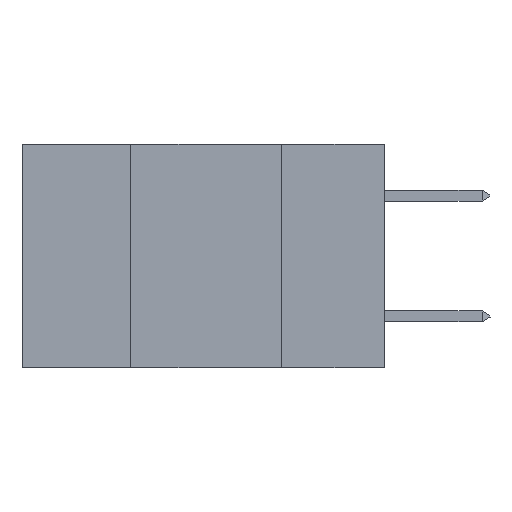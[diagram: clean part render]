
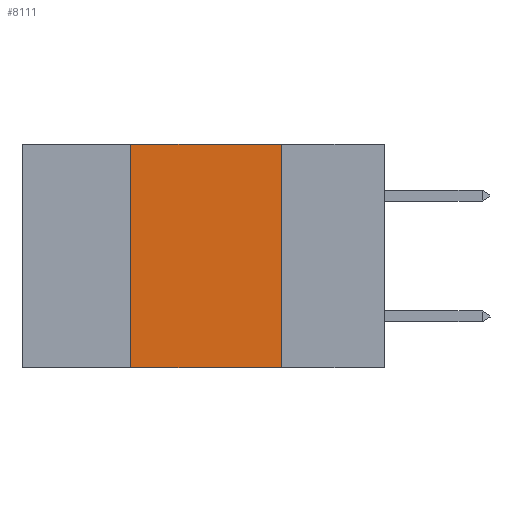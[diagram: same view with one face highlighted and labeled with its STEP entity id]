
A CAD part, left-side view. The second image highlights one B-rep face of the part: STEP entity #8111.
In plain terms, the highlighted planar face has unit normal (-1, 0, 0).
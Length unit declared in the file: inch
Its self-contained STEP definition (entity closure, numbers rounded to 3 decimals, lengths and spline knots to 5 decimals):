
#73 = CARTESIAN_POINT ( 'NONE',  ( 0., 0.17, 0. ) ) ;
#305 = ORIENTED_EDGE ( 'NONE', *, *, #475, .T. ) ;
#368 = CARTESIAN_POINT ( 'NONE',  ( 0., 0.17, 0. ) ) ;
#475 = EDGE_CURVE ( 'NONE', #9126, #8921, #4861, .T. ) ;
#551 = DIRECTION ( 'NONE',  ( 0., 0., 1. ) ) ;
#1289 = CARTESIAN_POINT ( 'NONE',  ( 0., 0.42, 0. ) ) ;
#1982 = DIRECTION ( 'NONE',  ( 0., 0., -1. ) ) ;
#2346 = VECTOR ( 'NONE', #6674, 39.37008 ) ;
#2566 = VERTEX_POINT ( 'NONE', #73 ) ;
#2651 = FACE_OUTER_BOUND ( 'NONE', #8831, .T. ) ;
#2859 = VECTOR ( 'NONE', #6045, 39.37008 ) ;
#3199 = EDGE_CURVE ( 'NONE', #8627, #2566, #7569, .T. ) ;
#3342 = CARTESIAN_POINT ( 'NONE',  ( 0., 0.42, 0. ) ) ;
#3367 = CARTESIAN_POINT ( 'NONE',  ( 0., 0.6, 0. ) ) ;
#3397 = DIRECTION ( 'NONE',  ( 0., -1., 0. ) ) ;
#4136 = LINE ( 'NONE', #368, #2346 ) ;
#4178 = EDGE_CURVE ( 'NONE', #9126, #8627, #5883, .T. ) ;
#4861 = LINE ( 'NONE', #6142, #2859 ) ;
#5614 = ORIENTED_EDGE ( 'NONE', *, *, #3199, .F. ) ;
#5883 = LINE ( 'NONE', #3342, #7784 ) ;
#6045 = DIRECTION ( 'NONE',  ( 0., -1., 0. ) ) ;
#6074 = DIRECTION ( 'NONE',  ( 1., 0., 0. ) ) ;
#6142 = CARTESIAN_POINT ( 'NONE',  ( 0., 0.6, -0.37 ) ) ;
#6674 = DIRECTION ( 'NONE',  ( 0., 0., -1. ) ) ;
#6719 = ORIENTED_EDGE ( 'NONE', *, *, #4178, .F. ) ;
#6848 = CARTESIAN_POINT ( 'NONE',  ( 0., 0.42, -0.37 ) ) ;
#7265 = CARTESIAN_POINT ( 'NONE',  ( 0., 0.17, -0.37 ) ) ;
#7354 = VECTOR ( 'NONE', #3397, 39.37008 ) ;
#7399 = AXIS2_PLACEMENT_3D ( 'NONE', #3367, #6074, #1982 ) ;
#7401 = ORIENTED_EDGE ( 'NONE', *, *, #7618, .F. ) ;
#7503 = CARTESIAN_POINT ( 'NONE',  ( 0., 0.6, 0. ) ) ;
#7569 = LINE ( 'NONE', #7503, #7354 ) ;
#7618 = EDGE_CURVE ( 'NONE', #2566, #8921, #4136, .T. ) ;
#7784 = VECTOR ( 'NONE', #551, 39.37008 ) ;
#8111 = ADVANCED_FACE ( 'NONE', ( #2651 ), #8992, .F. ) ;
#8627 = VERTEX_POINT ( 'NONE', #1289 ) ;
#8831 = EDGE_LOOP ( 'NONE', ( #7401, #5614, #6719, #305 ) ) ;
#8921 = VERTEX_POINT ( 'NONE', #7265 ) ;
#8992 = PLANE ( 'NONE',  #7399 ) ;
#9126 = VERTEX_POINT ( 'NONE', #6848 ) ;
